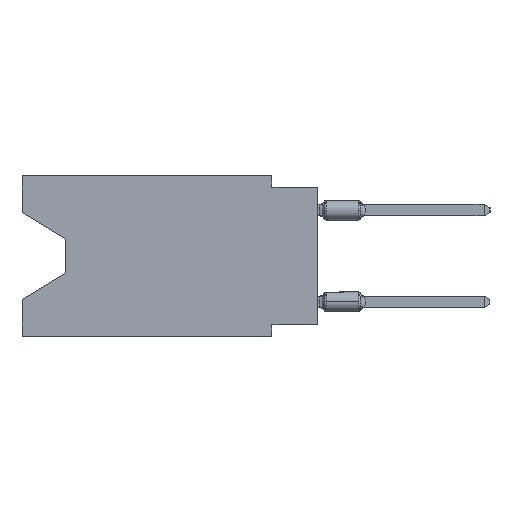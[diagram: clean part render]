
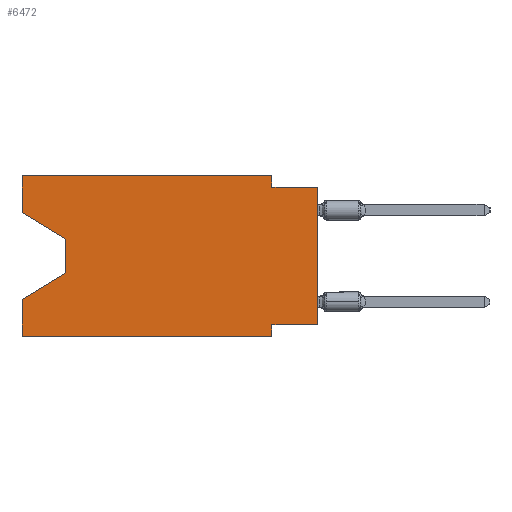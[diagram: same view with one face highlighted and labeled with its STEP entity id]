
A CAD part, left-side view. The second image highlights one B-rep face of the part: STEP entity #6472.
In plain terms, the highlighted planar face has unit normal (-1, 0, 0).
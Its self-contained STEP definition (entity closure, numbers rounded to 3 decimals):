
#1084 = FACE_OUTER_BOUND ( 'NONE', #6415, .T. ) ;
#1277 = DIRECTION ( 'NONE',  ( 0., 0., -1. ) ) ;
#1447 = LINE ( 'NONE', #15010, #26602 ) ;
#2052 = LINE ( 'NONE', #29362, #15127 ) ;
#2083 = ORIENTED_EDGE ( 'NONE', *, *, #23592, .T. ) ;
#2884 = LINE ( 'NONE', #13752, #29516 ) ;
#4199 = LINE ( 'NONE', #15233, #27301 ) ;
#4549 = EDGE_CURVE ( 'NONE', #21370, #11700, #33889, .T. ) ;
#5332 = CARTESIAN_POINT ( 'NONE',  ( 0., 13.97, -5.385 ) ) ;
#5996 = EDGE_CURVE ( 'NONE', #24807, #11087, #33516, .T. ) ;
#6164 = CARTESIAN_POINT ( 'NONE',  ( 0., 0., 0. ) ) ;
#6415 = EDGE_LOOP ( 'NONE', ( #31441, #23391, #17433, #11289, #2083, #29262, #25594, #28889, #24193, #23394, #23402, #32523 ) ) ;
#6472 = ADVANCED_FACE ( 'NONE', ( #1084 ), #31122, .F. ) ;
#6822 = CARTESIAN_POINT ( 'NONE',  ( 0., 16.383, 0. ) ) ;
#7479 = DIRECTION ( 'NONE',  ( 0., 0.855, -0.519 ) ) ;
#8502 = DIRECTION ( 'NONE',  ( 0., -1., 0. ) ) ;
#9115 = CARTESIAN_POINT ( 'NONE',  ( 0., 13.97, -3.505 ) ) ;
#9173 = VECTOR ( 'NONE', #17888, 1000. ) ;
#9441 = LINE ( 'NONE', #15026, #33796 ) ;
#9471 = DIRECTION ( 'NONE',  ( 0., 0., -1. ) ) ;
#9560 = EDGE_CURVE ( 'NONE', #12945, #29003, #9441, .T. ) ;
#9727 = DIRECTION ( 'NONE',  ( 0., 0., -1. ) ) ;
#10063 = CARTESIAN_POINT ( 'NONE',  ( 0., 16.383, -6.852 ) ) ;
#10367 = VERTEX_POINT ( 'NONE', #28973 ) ;
#11087 = VERTEX_POINT ( 'NONE', #6822 ) ;
#11289 = ORIENTED_EDGE ( 'NONE', *, *, #9560, .F. ) ;
#11575 = LINE ( 'NONE', #6164, #15594 ) ;
#11700 = VERTEX_POINT ( 'NONE', #5332 ) ;
#12410 = EDGE_CURVE ( 'NONE', #17019, #32296, #18573, .T. ) ;
#12477 = CARTESIAN_POINT ( 'NONE',  ( 0., 16.383, 0. ) ) ;
#12556 = CARTESIAN_POINT ( 'NONE',  ( 0., 2.54, -8.89 ) ) ;
#12945 = VERTEX_POINT ( 'NONE', #19069 ) ;
#13752 = CARTESIAN_POINT ( 'NONE',  ( 0., 16.383, -8.89 ) ) ;
#14035 = CARTESIAN_POINT ( 'NONE',  ( 0., 0., -8.255 ) ) ;
#14787 = CARTESIAN_POINT ( 'NONE',  ( 0., 2.54, 0. ) ) ;
#14919 = LINE ( 'NONE', #25943, #19391 ) ;
#14948 = VECTOR ( 'NONE', #1277, 1000. ) ;
#15010 = CARTESIAN_POINT ( 'NONE',  ( 0., 16.383, 0. ) ) ;
#15026 = CARTESIAN_POINT ( 'NONE',  ( 0., 16.383, 0. ) ) ;
#15127 = VECTOR ( 'NONE', #7479, 1000. ) ;
#15233 = CARTESIAN_POINT ( 'NONE',  ( 0., 16.383, -2.038 ) ) ;
#15326 = AXIS2_PLACEMENT_3D ( 'NONE', #17724, #22972, #20431 ) ;
#15594 = VECTOR ( 'NONE', #28046, 1000. ) ;
#15641 = EDGE_CURVE ( 'NONE', #10367, #24144, #14919, .T. ) ;
#16819 = CARTESIAN_POINT ( 'NONE',  ( 0., 16.383, -2.038 ) ) ;
#17019 = VERTEX_POINT ( 'NONE', #25912 ) ;
#17433 = ORIENTED_EDGE ( 'NONE', *, *, #32351, .T. ) ;
#17724 = CARTESIAN_POINT ( 'NONE',  ( 0., 16.383, 0. ) ) ;
#17888 = DIRECTION ( 'NONE',  ( 0., 0., 1. ) ) ;
#18573 = LINE ( 'NONE', #29622, #23239 ) ;
#18611 = EDGE_CURVE ( 'NONE', #24807, #21370, #4199, .T. ) ;
#19069 = CARTESIAN_POINT ( 'NONE',  ( 0., 16.383, -8.89 ) ) ;
#19391 = VECTOR ( 'NONE', #23241, 1000. ) ;
#20431 = DIRECTION ( 'NONE',  ( 0., 0., -1. ) ) ;
#20492 = VERTEX_POINT ( 'NONE', #14787 ) ;
#21370 = VERTEX_POINT ( 'NONE', #23135 ) ;
#22777 = VERTEX_POINT ( 'NONE', #33531 ) ;
#22972 = DIRECTION ( 'NONE',  ( 1., 0., 0. ) ) ;
#23135 = CARTESIAN_POINT ( 'NONE',  ( 0., 13.97, -3.505 ) ) ;
#23239 = VECTOR ( 'NONE', #9727, 1000. ) ;
#23241 = DIRECTION ( 'NONE',  ( 0., -1., 0. ) ) ;
#23391 = ORIENTED_EDGE ( 'NONE', *, *, #4549, .T. ) ;
#23394 = ORIENTED_EDGE ( 'NONE', *, *, #27425, .F. ) ;
#23402 = ORIENTED_EDGE ( 'NONE', *, *, #26158, .F. ) ;
#23592 = EDGE_CURVE ( 'NONE', #12945, #32296, #2884, .T. ) ;
#24144 = VERTEX_POINT ( 'NONE', #26104 ) ;
#24193 = ORIENTED_EDGE ( 'NONE', *, *, #15641, .F. ) ;
#24807 = VERTEX_POINT ( 'NONE', #16819 ) ;
#25093 = DIRECTION ( 'NONE',  ( 0., 0., 1. ) ) ;
#25594 = ORIENTED_EDGE ( 'NONE', *, *, #32006, .F. ) ;
#25912 = CARTESIAN_POINT ( 'NONE',  ( 0., 2.54, -8.255 ) ) ;
#25943 = CARTESIAN_POINT ( 'NONE',  ( 0., 0., -0.635 ) ) ;
#26031 = DIRECTION ( 'NONE',  ( 0., -1., 0. ) ) ;
#26104 = CARTESIAN_POINT ( 'NONE',  ( 0., 0., -0.635 ) ) ;
#26158 = EDGE_CURVE ( 'NONE', #11087, #20492, #1447, .T. ) ;
#26251 = DIRECTION ( 'NONE',  ( 0., -0.855, -0.519 ) ) ;
#26602 = VECTOR ( 'NONE', #26031, 1000. ) ;
#26981 = VECTOR ( 'NONE', #9471, 1000. ) ;
#27301 = VECTOR ( 'NONE', #26251, 1000. ) ;
#27416 = LINE ( 'NONE', #14035, #33596 ) ;
#27425 = EDGE_CURVE ( 'NONE', #20492, #10367, #30640, .T. ) ;
#27957 = DIRECTION ( 'NONE',  ( 0., 1., 0. ) ) ;
#28046 = DIRECTION ( 'NONE',  ( 0., 0., 1. ) ) ;
#28889 = ORIENTED_EDGE ( 'NONE', *, *, #34260, .T. ) ;
#28973 = CARTESIAN_POINT ( 'NONE',  ( 0., 2.54, -0.635 ) ) ;
#29003 = VERTEX_POINT ( 'NONE', #10063 ) ;
#29262 = ORIENTED_EDGE ( 'NONE', *, *, #12410, .F. ) ;
#29362 = CARTESIAN_POINT ( 'NONE',  ( 0., 13.97, -5.385 ) ) ;
#29516 = VECTOR ( 'NONE', #8502, 1000. ) ;
#29622 = CARTESIAN_POINT ( 'NONE',  ( 0., 2.54, -8.89 ) ) ;
#30640 = LINE ( 'NONE', #34197, #14948 ) ;
#31122 = PLANE ( 'NONE',  #15326 ) ;
#31441 = ORIENTED_EDGE ( 'NONE', *, *, #18611, .T. ) ;
#32006 = EDGE_CURVE ( 'NONE', #22777, #17019, #27416, .T. ) ;
#32296 = VERTEX_POINT ( 'NONE', #12556 ) ;
#32351 = EDGE_CURVE ( 'NONE', #11700, #29003, #2052, .T. ) ;
#32523 = ORIENTED_EDGE ( 'NONE', *, *, #5996, .F. ) ;
#33516 = LINE ( 'NONE', #12477, #9173 ) ;
#33531 = CARTESIAN_POINT ( 'NONE',  ( 0., 0., -8.255 ) ) ;
#33596 = VECTOR ( 'NONE', #27957, 1000. ) ;
#33796 = VECTOR ( 'NONE', #25093, 1000. ) ;
#33889 = LINE ( 'NONE', #9115, #26981 ) ;
#34197 = CARTESIAN_POINT ( 'NONE',  ( 0., 2.54, 0. ) ) ;
#34260 = EDGE_CURVE ( 'NONE', #22777, #24144, #11575, .T. ) ;
